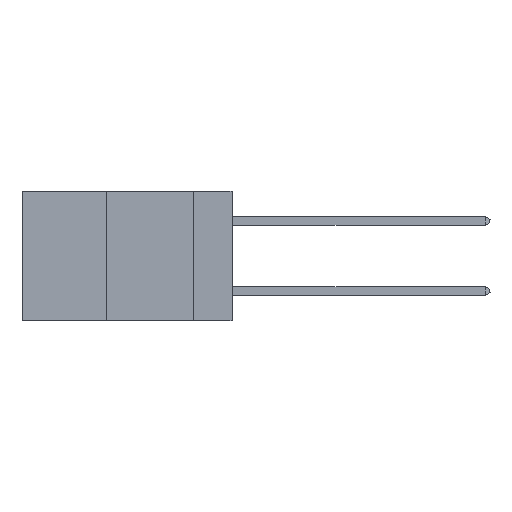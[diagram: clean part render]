
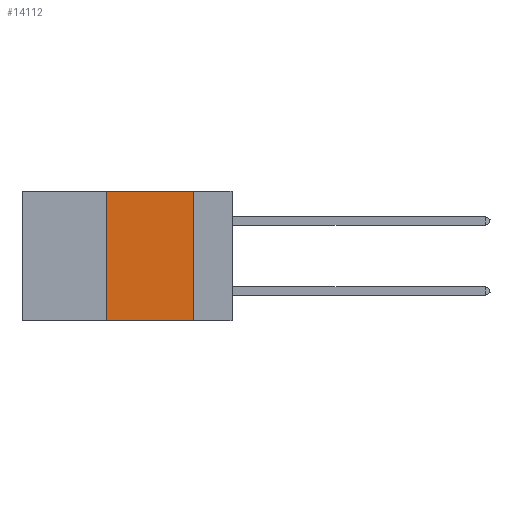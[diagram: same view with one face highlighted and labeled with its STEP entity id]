
A CAD part, left-side view. The second image highlights one B-rep face of the part: STEP entity #14112.
In plain terms, the highlighted planar face has unit normal (-1, 0, 0).
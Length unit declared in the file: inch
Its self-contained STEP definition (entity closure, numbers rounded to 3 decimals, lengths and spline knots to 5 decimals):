
#491 = AXIS2_PLACEMENT_3D ( 'NONE', #18070, #4721, #41976 ) ;
#1230 = EDGE_CURVE ( 'NONE', #43592, #38645, #10124, .T. ) ;
#1616 = VERTEX_POINT ( 'NONE', #4002 ) ;
#1932 = LINE ( 'NONE', #24624, #6195 ) ;
#2473 = DIRECTION ( 'NONE',  ( 0., -1., 0. ) ) ;
#4002 = CARTESIAN_POINT ( 'NONE',  ( 0., 0.36, 0. ) ) ;
#4721 = DIRECTION ( 'NONE',  ( 1., 0., 0. ) ) ;
#5750 = CARTESIAN_POINT ( 'NONE',  ( 0., 0.36, -0.37 ) ) ;
#6195 = VECTOR ( 'NONE', #37812, 39.37008 ) ;
#8326 = PLANE ( 'NONE',  #491 ) ;
#8381 = ORIENTED_EDGE ( 'NONE', *, *, #38038, .F. ) ;
#10124 = LINE ( 'NONE', #43344, #13788 ) ;
#12877 = CARTESIAN_POINT ( 'NONE',  ( 0., 0.6, 0. ) ) ;
#13788 = VECTOR ( 'NONE', #43488, 39.37008 ) ;
#14112 = ADVANCED_FACE ( 'NONE', ( #34514 ), #8326, .F. ) ;
#14979 = ORIENTED_EDGE ( 'NONE', *, *, #21104, .F. ) ;
#15219 = ORIENTED_EDGE ( 'NONE', *, *, #1230, .T. ) ;
#15979 = CARTESIAN_POINT ( 'NONE',  ( 0., 0.11, 0. ) ) ;
#18070 = CARTESIAN_POINT ( 'NONE',  ( 0., 0.6, 0. ) ) ;
#18359 = VECTOR ( 'NONE', #2473, 39.37008 ) ;
#19338 = LINE ( 'NONE', #30857, #33171 ) ;
#20345 = CARTESIAN_POINT ( 'NONE',  ( 0., 0.11, -0.37 ) ) ;
#21104 = EDGE_CURVE ( 'NONE', #43592, #1616, #19338, .T. ) ;
#21479 = ORIENTED_EDGE ( 'NONE', *, *, #37563, .F. ) ;
#23729 = DIRECTION ( 'NONE',  ( 0., 0., 1. ) ) ;
#24624 = CARTESIAN_POINT ( 'NONE',  ( 0., 0.11, 0. ) ) ;
#30857 = CARTESIAN_POINT ( 'NONE',  ( 0., 0.36, 0. ) ) ;
#33171 = VECTOR ( 'NONE', #23729, 39.37008 ) ;
#34514 = FACE_OUTER_BOUND ( 'NONE', #42527, .T. ) ;
#36847 = VERTEX_POINT ( 'NONE', #15979 ) ;
#36937 = LINE ( 'NONE', #12877, #18359 ) ;
#37563 = EDGE_CURVE ( 'NONE', #36847, #38645, #1932, .T. ) ;
#37812 = DIRECTION ( 'NONE',  ( 0., 0., -1. ) ) ;
#38038 = EDGE_CURVE ( 'NONE', #1616, #36847, #36937, .T. ) ;
#38645 = VERTEX_POINT ( 'NONE', #20345 ) ;
#41976 = DIRECTION ( 'NONE',  ( 0., 0., -1. ) ) ;
#42527 = EDGE_LOOP ( 'NONE', ( #21479, #8381, #14979, #15219 ) ) ;
#43344 = CARTESIAN_POINT ( 'NONE',  ( 0., 0.6, -0.37 ) ) ;
#43488 = DIRECTION ( 'NONE',  ( 0., -1., 0. ) ) ;
#43592 = VERTEX_POINT ( 'NONE', #5750 ) ;
